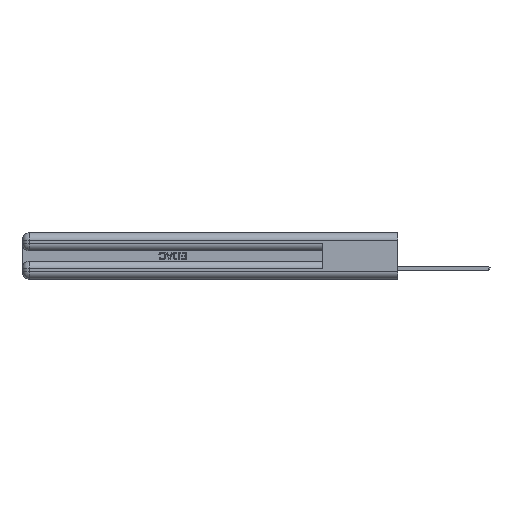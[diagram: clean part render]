
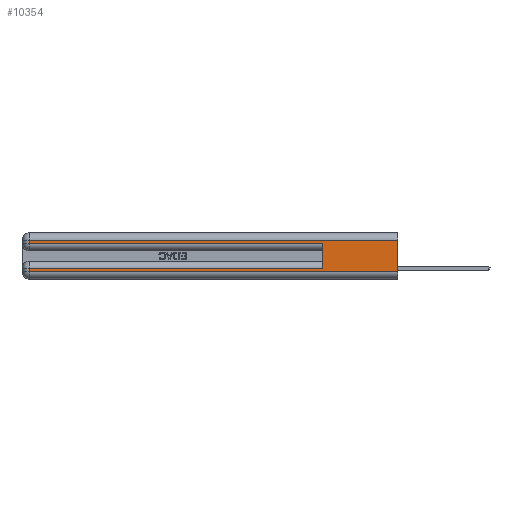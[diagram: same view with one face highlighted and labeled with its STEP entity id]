
A CAD part, left-side view. The second image highlights one B-rep face of the part: STEP entity #10354.
In plain terms, the highlighted planar face has unit normal (-1, 0, 0).
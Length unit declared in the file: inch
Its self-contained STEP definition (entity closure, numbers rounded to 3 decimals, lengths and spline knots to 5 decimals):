
#97 = CARTESIAN_POINT ( 'NONE',  ( 0., 0., 0.285 ) ) ;
#989 = CARTESIAN_POINT ( 'NONE',  ( 0., 0., 0.085 ) ) ;
#1656 = CARTESIAN_POINT ( 'NONE',  ( 0., 2.94, 0.31 ) ) ;
#2565 = VERTEX_POINT ( 'NONE', #8736 ) ;
#2589 = CARTESIAN_POINT ( 'NONE',  ( 0., 2.94, 0.285 ) ) ;
#4218 = EDGE_CURVE ( 'NONE', #11701, #2565, #15960, .T. ) ;
#4982 = CARTESIAN_POINT ( 'NONE',  ( 0., 2.94, 0.085 ) ) ;
#5046 = DIRECTION ( 'NONE',  ( 0., 1., 0. ) ) ;
#5105 = VECTOR ( 'NONE', #29760, 39.37008 ) ;
#5465 = LINE ( 'NONE', #989, #29899 ) ;
#6188 = VECTOR ( 'NONE', #5046, 39.37008 ) ;
#6781 = VECTOR ( 'NONE', #8558, 39.37008 ) ;
#7936 = ORIENTED_EDGE ( 'NONE', *, *, #40878, .F. ) ;
#7975 = VERTEX_POINT ( 'NONE', #2589 ) ;
#8558 = DIRECTION ( 'NONE',  ( 0., -1., 0. ) ) ;
#8736 = CARTESIAN_POINT ( 'NONE',  ( 0., 0., 0.06 ) ) ;
#8859 = EDGE_LOOP ( 'NONE', ( #7936, #46220, #38827, #39208, #44123, #36581, #16394, #18102 ) ) ;
#10354 = ADVANCED_FACE ( 'NONE', ( #13380 ), #26746, .F. ) ;
#11701 = VERTEX_POINT ( 'NONE', #44981 ) ;
#12657 = EDGE_CURVE ( 'NONE', #43376, #48456, #5465, .T. ) ;
#13380 = FACE_OUTER_BOUND ( 'NONE', #8859, .T. ) ;
#13557 = VECTOR ( 'NONE', #53090, 39.37008 ) ;
#14871 = VERTEX_POINT ( 'NONE', #51698 ) ;
#15529 = CARTESIAN_POINT ( 'NONE',  ( 0., 2.94, 0.37 ) ) ;
#15960 = LINE ( 'NONE', #38704, #5105 ) ;
#16394 = ORIENTED_EDGE ( 'NONE', *, *, #25849, .T. ) ;
#16988 = CARTESIAN_POINT ( 'NONE',  ( 0., 0.6, 0.285 ) ) ;
#17446 = CARTESIAN_POINT ( 'NONE',  ( 0., 0.6, 0.145 ) ) ;
#17518 = CARTESIAN_POINT ( 'NONE',  ( 0., 0., 0.31 ) ) ;
#18102 = ORIENTED_EDGE ( 'NONE', *, *, #4218, .T. ) ;
#19778 = LINE ( 'NONE', #36996, #25612 ) ;
#20932 = LINE ( 'NONE', #17518, #6188 ) ;
#22221 = CARTESIAN_POINT ( 'NONE',  ( 0., 0., 0.37 ) ) ;
#22392 = DIRECTION ( 'NONE',  ( 0., 0., -1. ) ) ;
#24013 = DIRECTION ( 'NONE',  ( 0., 0., -1. ) ) ;
#25612 = VECTOR ( 'NONE', #41303, 39.37008 ) ;
#25671 = VECTOR ( 'NONE', #24013, 39.37008 ) ;
#25849 = EDGE_CURVE ( 'NONE', #48456, #11701, #46433, .T. ) ;
#26507 = VECTOR ( 'NONE', #29736, 39.37008 ) ;
#26746 = PLANE ( 'NONE',  #32893 ) ;
#27348 = LINE ( 'NONE', #97, #6781 ) ;
#29731 = DIRECTION ( 'NONE',  ( 0., 1., 0. ) ) ;
#29736 = DIRECTION ( 'NONE',  ( 0., 0., 1. ) ) ;
#29760 = DIRECTION ( 'NONE',  ( 0., -1., 0. ) ) ;
#29899 = VECTOR ( 'NONE', #29731, 39.37008 ) ;
#31970 = EDGE_CURVE ( 'NONE', #14871, #47317, #20932, .T. ) ;
#32893 = AXIS2_PLACEMENT_3D ( 'NONE', #22221, #51029, #22392 ) ;
#34314 = CARTESIAN_POINT ( 'NONE',  ( 0., 0.6, 0.085 ) ) ;
#36581 = ORIENTED_EDGE ( 'NONE', *, *, #12657, .T. ) ;
#36996 = CARTESIAN_POINT ( 'NONE',  ( 0., 0., 0.37 ) ) ;
#38704 = CARTESIAN_POINT ( 'NONE',  ( 0., 0., 0.06 ) ) ;
#38827 = ORIENTED_EDGE ( 'NONE', *, *, #41135, .T. ) ;
#39208 = ORIENTED_EDGE ( 'NONE', *, *, #48272, .T. ) ;
#40677 = CARTESIAN_POINT ( 'NONE',  ( 0., 2.94, 0.37 ) ) ;
#40878 = EDGE_CURVE ( 'NONE', #14871, #2565, #19778, .T. ) ;
#41135 = EDGE_CURVE ( 'NONE', #47317, #7975, #48876, .T. ) ;
#41303 = DIRECTION ( 'NONE',  ( 0., 0., -1. ) ) ;
#43376 = VERTEX_POINT ( 'NONE', #34314 ) ;
#44123 = ORIENTED_EDGE ( 'NONE', *, *, #49913, .F. ) ;
#44981 = CARTESIAN_POINT ( 'NONE',  ( 0., 2.94, 0.06 ) ) ;
#46220 = ORIENTED_EDGE ( 'NONE', *, *, #31970, .T. ) ;
#46433 = LINE ( 'NONE', #40677, #13557 ) ;
#47317 = VERTEX_POINT ( 'NONE', #1656 ) ;
#47791 = LINE ( 'NONE', #17446, #26507 ) ;
#48272 = EDGE_CURVE ( 'NONE', #7975, #52112, #27348, .T. ) ;
#48456 = VERTEX_POINT ( 'NONE', #4982 ) ;
#48876 = LINE ( 'NONE', #15529, #25671 ) ;
#49913 = EDGE_CURVE ( 'NONE', #43376, #52112, #47791, .T. ) ;
#51029 = DIRECTION ( 'NONE',  ( 1., 0., 0. ) ) ;
#51698 = CARTESIAN_POINT ( 'NONE',  ( 0., 0., 0.31 ) ) ;
#52112 = VERTEX_POINT ( 'NONE', #16988 ) ;
#53090 = DIRECTION ( 'NONE',  ( 0., 0., -1. ) ) ;
